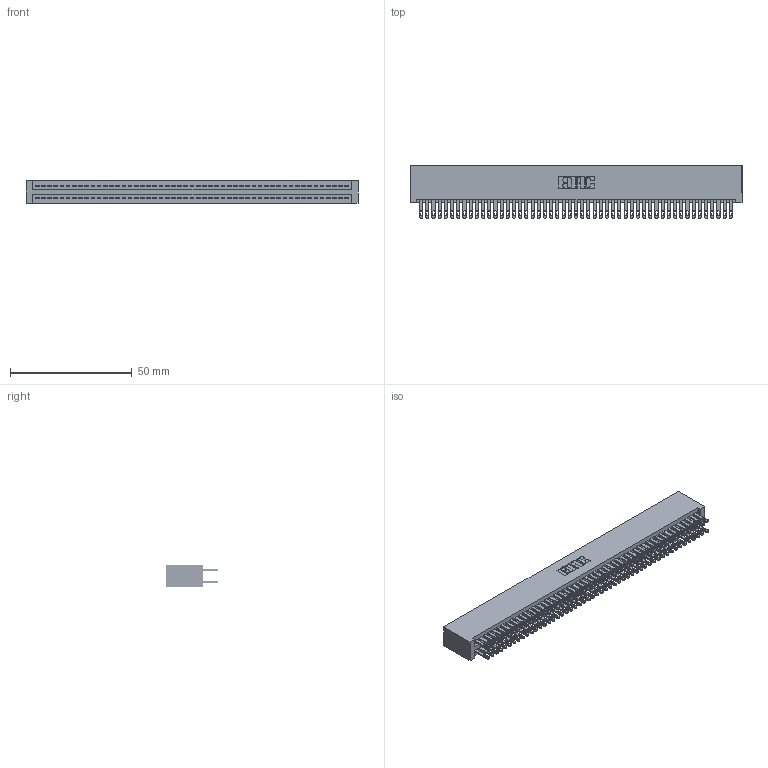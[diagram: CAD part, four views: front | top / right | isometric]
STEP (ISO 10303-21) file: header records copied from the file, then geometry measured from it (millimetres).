
FILE_DESCRIPTION (( 'STEP AP203' ), '1' );
FILE_NAME ('345-102-500-201.STEP', '2018-10-05T18:19:02', ( '' ), ( '' ), 'SwSTEP 2.0', 'SolidWorks 2016', '' );
FILE_SCHEMA (( 'CONFIG_CONTROL_DESIGN' ));
Length unit declared in the file: inch
Products named in the file (3): 345-292-001_345-293-100; 345-102-500-201; 345 Part_No Mounting Lugs
Assembly tree (103 placements, depth 2):
  345-102-500-201
    345 Part_No Mounting Lugs
    345-292-001_345-293-100  x102
Bounding box: 136.14 x 21.51 x 9.4 mm (x, y, z)
Volume: 14236.3 mm3; surface area: 22561.6 mm2
Topology: 103 solids, 103 shells, 4810 faces, 14699 edges, 9798 vertices
Faces by surface type: plane 2830, cylinder 1980
Entity records: 38457 total; most frequent: CARTESIAN_POINT 6436, ORIENTED_EDGE 6370, DIRECTION 5661, EDGE_CURVE 3185, LINE 2853, VECTOR 2853, VERTEX_POINT 2122, AXIS2_PLACEMENT_3D 1404
